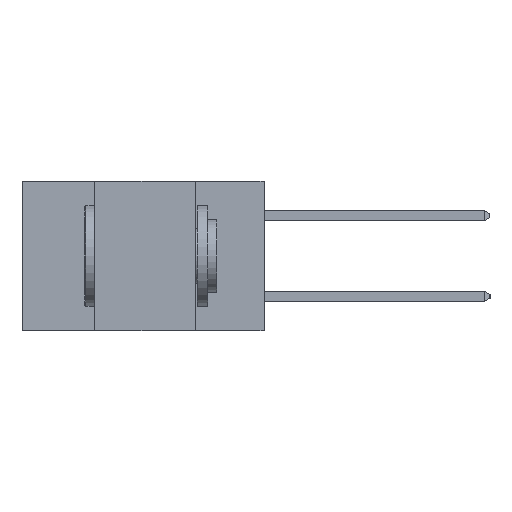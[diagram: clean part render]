
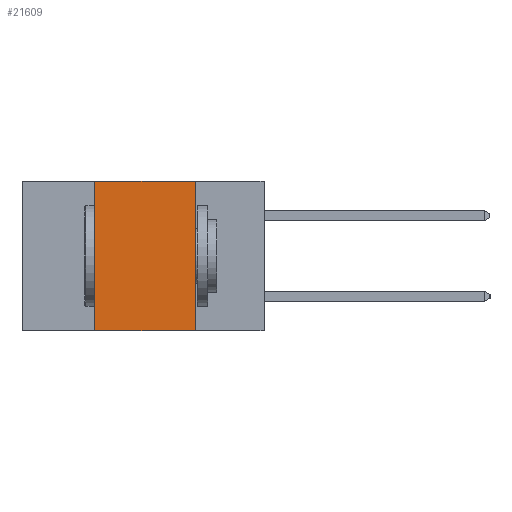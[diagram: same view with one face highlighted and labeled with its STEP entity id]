
A CAD part, left-side view. The second image highlights one B-rep face of the part: STEP entity #21609.
In plain terms, the highlighted planar face has unit normal (-1, 0, 0).
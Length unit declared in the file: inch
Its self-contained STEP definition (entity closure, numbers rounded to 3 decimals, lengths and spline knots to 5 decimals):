
#245 = ORIENTED_EDGE ( 'NONE', *, *, #11239, .F. ) ;
#417 = EDGE_CURVE ( 'NONE', #4652, #21833, #20657, .T. ) ;
#2060 = VECTOR ( 'NONE', #16107, 39.37008 ) ;
#2495 = VERTEX_POINT ( 'NONE', #15431 ) ;
#4652 = VERTEX_POINT ( 'NONE', #4807 ) ;
#4807 = CARTESIAN_POINT ( 'NONE',  ( 0., 0.42, 0. ) ) ;
#5000 = PLANE ( 'NONE',  #14753 ) ;
#6716 = DIRECTION ( 'NONE',  ( 0., -1., 0. ) ) ;
#6803 = DIRECTION ( 'NONE',  ( 1., 0., 0. ) ) ;
#8223 = ORIENTED_EDGE ( 'NONE', *, *, #21571, .T. ) ;
#8403 = DIRECTION ( 'NONE',  ( 0., 0., -1. ) ) ;
#8904 = VECTOR ( 'NONE', #8403, 39.37008 ) ;
#9466 = LINE ( 'NONE', #17060, #8904 ) ;
#10972 = VECTOR ( 'NONE', #19689, 39.37008 ) ;
#11239 = EDGE_CURVE ( 'NONE', #21833, #2495, #9466, .T. ) ;
#11543 = LINE ( 'NONE', #14373, #2060 ) ;
#13447 = VERTEX_POINT ( 'NONE', #20856 ) ;
#13506 = VECTOR ( 'NONE', #6716, 39.37008 ) ;
#13892 = ORIENTED_EDGE ( 'NONE', *, *, #417, .F. ) ;
#14373 = CARTESIAN_POINT ( 'NONE',  ( 0., 0.42, -0.37 ) ) ;
#14395 = CARTESIAN_POINT ( 'NONE',  ( 0., 0.17, 0. ) ) ;
#14753 = AXIS2_PLACEMENT_3D ( 'NONE', #17245, #6803, #18948 ) ;
#15431 = CARTESIAN_POINT ( 'NONE',  ( 0., 0.17, -0.37 ) ) ;
#15468 = CARTESIAN_POINT ( 'NONE',  ( 0., 0.6, -0.37 ) ) ;
#16107 = DIRECTION ( 'NONE',  ( 0., 0., 1. ) ) ;
#16968 = EDGE_LOOP ( 'NONE', ( #245, #13892, #17779, #8223 ) ) ;
#17060 = CARTESIAN_POINT ( 'NONE',  ( 0., 0.17, -0.37 ) ) ;
#17245 = CARTESIAN_POINT ( 'NONE',  ( 0., 0.6, 0. ) ) ;
#17779 = ORIENTED_EDGE ( 'NONE', *, *, #20471, .F. ) ;
#18330 = CARTESIAN_POINT ( 'NONE',  ( 0., 0.6, 0. ) ) ;
#18584 = LINE ( 'NONE', #15468, #13506 ) ;
#18948 = DIRECTION ( 'NONE',  ( 0., 0., -1. ) ) ;
#19689 = DIRECTION ( 'NONE',  ( 0., -1., 0. ) ) ;
#20471 = EDGE_CURVE ( 'NONE', #13447, #4652, #11543, .T. ) ;
#20657 = LINE ( 'NONE', #18330, #10972 ) ;
#20856 = CARTESIAN_POINT ( 'NONE',  ( 0., 0.42, -0.37 ) ) ;
#21571 = EDGE_CURVE ( 'NONE', #13447, #2495, #18584, .T. ) ;
#21609 = ADVANCED_FACE ( 'NONE', ( #22098 ), #5000, .F. ) ;
#21833 = VERTEX_POINT ( 'NONE', #14395 ) ;
#22098 = FACE_OUTER_BOUND ( 'NONE', #16968, .T. ) ;
